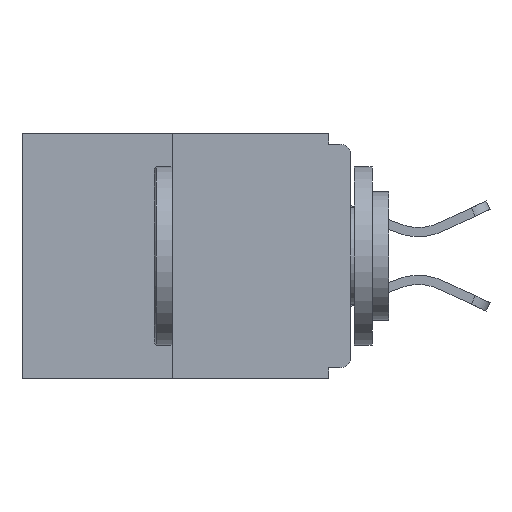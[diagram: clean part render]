
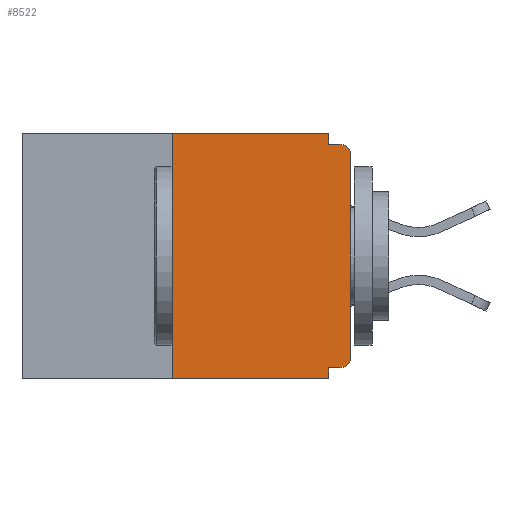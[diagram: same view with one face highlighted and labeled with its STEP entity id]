
A CAD part, left-side view. The second image highlights one B-rep face of the part: STEP entity #8522.
In plain terms, the highlighted planar face has unit normal (-1, 0, 0).
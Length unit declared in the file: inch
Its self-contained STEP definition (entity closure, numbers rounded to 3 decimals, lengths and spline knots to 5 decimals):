
#109 = CARTESIAN_POINT ( 'NONE',  ( 0., 0.25, -0.343 ) ) ;
#1109 = CARTESIAN_POINT ( 'NONE',  ( 0., 0., 0. ) ) ;
#1315 = CARTESIAN_POINT ( 'NONE',  ( 0., 0.031, 0. ) ) ;
#1317 = VECTOR ( 'NONE', #2969, 39.37008 ) ;
#1643 = EDGE_CURVE ( 'NONE', #28404, #18569, #13407, .T. ) ;
#1687 = PLANE ( 'NONE',  #1884 ) ;
#1702 = DIRECTION ( 'NONE',  ( 0., -1., 0. ) ) ;
#1802 = DIRECTION ( 'NONE',  ( 0., 0., -1. ) ) ;
#1884 = AXIS2_PLACEMENT_3D ( 'NONE', #2107, #22988, #1802 ) ;
#1990 = ORIENTED_EDGE ( 'NONE', *, *, #2606, .F. ) ;
#2107 = CARTESIAN_POINT ( 'NONE',  ( 0., 0.46, 0. ) ) ;
#2166 = VERTEX_POINT ( 'NONE', #27280 ) ;
#2450 = VECTOR ( 'NONE', #8861, 39.37008 ) ;
#2606 = EDGE_CURVE ( 'NONE', #2624, #29667, #8813, .T. ) ;
#2624 = VERTEX_POINT ( 'NONE', #1315 ) ;
#2752 = DIRECTION ( 'NONE',  ( 0., 1., 0. ) ) ;
#2969 = DIRECTION ( 'NONE',  ( 0., 0., 1. ) ) ;
#3120 = VECTOR ( 'NONE', #1702, 39.37008 ) ;
#3895 = CARTESIAN_POINT ( 'NONE',  ( 0., 0., -0.015 ) ) ;
#4218 = DIRECTION ( 'NONE',  ( -1., 0., 0. ) ) ;
#4346 = AXIS2_PLACEMENT_3D ( 'NONE', #6888, #4218, #25577 ) ;
#4522 = CARTESIAN_POINT ( 'NONE',  ( 0., 0.46, 0. ) ) ;
#4680 = EDGE_CURVE ( 'NONE', #2166, #25328, #7231, .T. ) ;
#5446 = VERTEX_POINT ( 'NONE', #109 ) ;
#6264 = FACE_OUTER_BOUND ( 'NONE', #12867, .T. ) ;
#6815 = CARTESIAN_POINT ( 'NONE',  ( 0., 0., -0.313 ) ) ;
#6888 = CARTESIAN_POINT ( 'NONE',  ( 0., 0.015, -0.313 ) ) ;
#7231 = LINE ( 'NONE', #9754, #11245 ) ;
#7497 = CARTESIAN_POINT ( 'NONE',  ( 0., 0.031, -0.328 ) ) ;
#7956 = DIRECTION ( 'NONE',  ( 0., -1., 0. ) ) ;
#8009 = LINE ( 'NONE', #1109, #29248 ) ;
#8522 = ADVANCED_FACE ( 'NONE', ( #6264 ), #1687, .F. ) ;
#8813 = LINE ( 'NONE', #15189, #27198 ) ;
#8818 = VECTOR ( 'NONE', #8893, 39.37008 ) ;
#8861 = DIRECTION ( 'NONE',  ( 0., -1., 0. ) ) ;
#8893 = DIRECTION ( 'NONE',  ( 0., 0., -1. ) ) ;
#9754 = CARTESIAN_POINT ( 'NONE',  ( 0., 0., -0.328 ) ) ;
#9757 = EDGE_CURVE ( 'NONE', #19434, #28404, #8009, .T. ) ;
#10222 = ORIENTED_EDGE ( 'NONE', *, *, #15577, .F. ) ;
#11245 = VECTOR ( 'NONE', #2752, 39.37008 ) ;
#12867 = EDGE_LOOP ( 'NONE', ( #23172, #15785, #30079, #25891, #18205, #20493, #15046, #16645, #10222, #1990 ) ) ;
#13407 = CIRCLE ( 'NONE', #29066, 0.015 ) ;
#13521 = VERTEX_POINT ( 'NONE', #22155 ) ;
#14096 = DIRECTION ( 'NONE',  ( -1., 0., 0. ) ) ;
#14542 = LINE ( 'NONE', #19245, #1317 ) ;
#15046 = ORIENTED_EDGE ( 'NONE', *, *, #9757, .T. ) ;
#15189 = CARTESIAN_POINT ( 'NONE',  ( 0., 0.031, 0. ) ) ;
#15577 = EDGE_CURVE ( 'NONE', #29667, #18569, #23368, .T. ) ;
#15785 = ORIENTED_EDGE ( 'NONE', *, *, #24019, .F. ) ;
#16198 = CARTESIAN_POINT ( 'NONE',  ( 0., 0.25, 0. ) ) ;
#16527 = LINE ( 'NONE', #29685, #8818 ) ;
#16645 = ORIENTED_EDGE ( 'NONE', *, *, #1643, .T. ) ;
#17080 = CARTESIAN_POINT ( 'NONE',  ( 0., 0.015, -0.015 ) ) ;
#17121 = CARTESIAN_POINT ( 'NONE',  ( 0., 0.031, -0.015 ) ) ;
#18205 = ORIENTED_EDGE ( 'NONE', *, *, #4680, .F. ) ;
#18569 = VERTEX_POINT ( 'NONE', #17080 ) ;
#19054 = DIRECTION ( 'NONE',  ( 0., 0., -1. ) ) ;
#19245 = CARTESIAN_POINT ( 'NONE',  ( 0., 0.25, 0. ) ) ;
#19434 = VERTEX_POINT ( 'NONE', #6815 ) ;
#19618 = CIRCLE ( 'NONE', #4346, 0.015 ) ;
#19890 = CARTESIAN_POINT ( 'NONE',  ( 0., 0.46, -0.343 ) ) ;
#20493 = ORIENTED_EDGE ( 'NONE', *, *, #25087, .T. ) ;
#21312 = EDGE_CURVE ( 'NONE', #25328, #13521, #16527, .T. ) ;
#22155 = CARTESIAN_POINT ( 'NONE',  ( 0., 0.031, -0.343 ) ) ;
#22988 = DIRECTION ( 'NONE',  ( 1., 0., 0. ) ) ;
#23172 = ORIENTED_EDGE ( 'NONE', *, *, #27839, .F. ) ;
#23331 = VECTOR ( 'NONE', #7956, 39.37008 ) ;
#23368 = LINE ( 'NONE', #3895, #3120 ) ;
#24019 = EDGE_CURVE ( 'NONE', #5446, #27200, #14542, .T. ) ;
#24222 = DIRECTION ( 'NONE',  ( 0., 0., -1. ) ) ;
#24667 = DIRECTION ( 'NONE',  ( 0., 0., 1. ) ) ;
#24810 = CARTESIAN_POINT ( 'NONE',  ( 0., 0., -0.03 ) ) ;
#25087 = EDGE_CURVE ( 'NONE', #2166, #19434, #19618, .T. ) ;
#25328 = VERTEX_POINT ( 'NONE', #7497 ) ;
#25577 = DIRECTION ( 'NONE',  ( 0., 0., -1. ) ) ;
#25891 = ORIENTED_EDGE ( 'NONE', *, *, #21312, .F. ) ;
#27198 = VECTOR ( 'NONE', #24222, 39.37008 ) ;
#27200 = VERTEX_POINT ( 'NONE', #16198 ) ;
#27280 = CARTESIAN_POINT ( 'NONE',  ( 0., 0.015, -0.328 ) ) ;
#27372 = LINE ( 'NONE', #19890, #23331 ) ;
#27839 = EDGE_CURVE ( 'NONE', #27200, #2624, #29963, .T. ) ;
#28277 = CARTESIAN_POINT ( 'NONE',  ( 0., 0.015, -0.03 ) ) ;
#28404 = VERTEX_POINT ( 'NONE', #24810 ) ;
#28991 = EDGE_CURVE ( 'NONE', #5446, #13521, #27372, .T. ) ;
#29066 = AXIS2_PLACEMENT_3D ( 'NONE', #28277, #14096, #19054 ) ;
#29248 = VECTOR ( 'NONE', #24667, 39.37008 ) ;
#29667 = VERTEX_POINT ( 'NONE', #17121 ) ;
#29685 = CARTESIAN_POINT ( 'NONE',  ( 0., 0.031, -0.343 ) ) ;
#29963 = LINE ( 'NONE', #4522, #2450 ) ;
#30079 = ORIENTED_EDGE ( 'NONE', *, *, #28991, .T. ) ;
